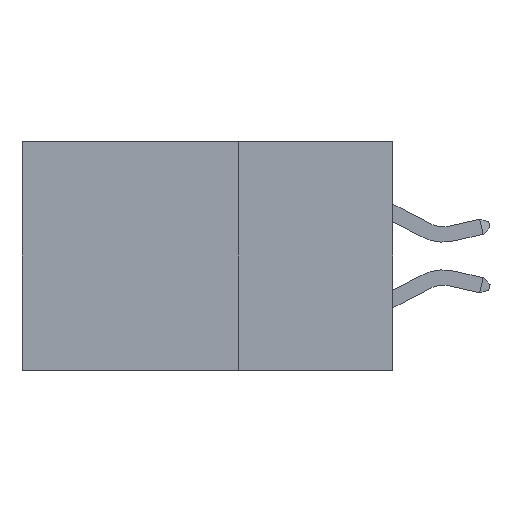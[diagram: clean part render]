
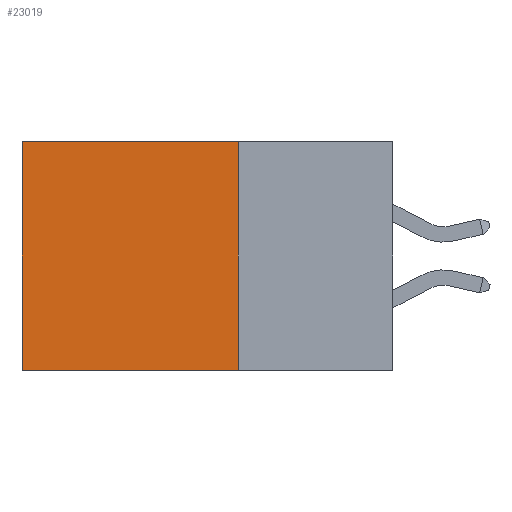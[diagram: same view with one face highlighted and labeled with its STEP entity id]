
A CAD part, left-side view. The second image highlights one B-rep face of the part: STEP entity #23019.
In plain terms, the highlighted planar face has unit normal (-1, 0, 0).
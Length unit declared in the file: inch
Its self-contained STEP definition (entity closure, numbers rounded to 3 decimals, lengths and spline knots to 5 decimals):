
#319 = CARTESIAN_POINT ( 'NONE',  ( 0.2875, 0.6, -0.37 ) ) ;
#680 = ORIENTED_EDGE ( 'NONE', *, *, #13594, .T. ) ;
#1024 = CARTESIAN_POINT ( 'NONE',  ( 0.2875, 0.25, 0. ) ) ;
#2021 = LINE ( 'NONE', #1024, #28720 ) ;
#2973 = EDGE_LOOP ( 'NONE', ( #680, #29762, #11356, #15714 ) ) ;
#3159 = VECTOR ( 'NONE', #13991, 39.37008 ) ;
#4450 = DIRECTION ( 'NONE',  ( 0., 1., 0. ) ) ;
#5563 = VERTEX_POINT ( 'NONE', #319 ) ;
#6186 = DIRECTION ( 'NONE',  ( 0., 0., -1. ) ) ;
#6781 = CARTESIAN_POINT ( 'NONE',  ( 0.2875, 0.25, -0.37 ) ) ;
#6893 = CARTESIAN_POINT ( 'NONE',  ( 0.2875, 0.25, -0.37 ) ) ;
#8074 = LINE ( 'NONE', #29714, #28807 ) ;
#8565 = CARTESIAN_POINT ( 'NONE',  ( 0.2875, 0.25, 0. ) ) ;
#8981 = VERTEX_POINT ( 'NONE', #8565 ) ;
#9592 = LINE ( 'NONE', #6893, #12648 ) ;
#9900 = PLANE ( 'NONE',  #10749 ) ;
#10749 = AXIS2_PLACEMENT_3D ( 'NONE', #19588, #26543, #12347 ) ;
#11356 = ORIENTED_EDGE ( 'NONE', *, *, #23941, .F. ) ;
#12347 = DIRECTION ( 'NONE',  ( 0., 0., -1. ) ) ;
#12648 = VECTOR ( 'NONE', #4450, 39.37008 ) ;
#12972 = FACE_OUTER_BOUND ( 'NONE', #2973, .T. ) ;
#13594 = EDGE_CURVE ( 'NONE', #27870, #5563, #16407, .T. ) ;
#13632 = EDGE_CURVE ( 'NONE', #14733, #5563, #9592, .T. ) ;
#13991 = DIRECTION ( 'NONE',  ( 0., 0., -1. ) ) ;
#14733 = VERTEX_POINT ( 'NONE', #6781 ) ;
#15714 = ORIENTED_EDGE ( 'NONE', *, *, #22500, .T. ) ;
#16407 = LINE ( 'NONE', #23647, #3159 ) ;
#19588 = CARTESIAN_POINT ( 'NONE',  ( 0.2875, 0.25, 0. ) ) ;
#22500 = EDGE_CURVE ( 'NONE', #8981, #27870, #8074, .T. ) ;
#23019 = ADVANCED_FACE ( 'NONE', ( #12972 ), #9900, .F. ) ;
#23647 = CARTESIAN_POINT ( 'NONE',  ( 0.2875, 0.6, 0. ) ) ;
#23941 = EDGE_CURVE ( 'NONE', #8981, #14733, #2021, .T. ) ;
#26543 = DIRECTION ( 'NONE',  ( 1., 0., 0. ) ) ;
#27870 = VERTEX_POINT ( 'NONE', #28608 ) ;
#28608 = CARTESIAN_POINT ( 'NONE',  ( 0.2875, 0.6, 0. ) ) ;
#28720 = VECTOR ( 'NONE', #6186, 39.37008 ) ;
#28807 = VECTOR ( 'NONE', #29819, 39.37008 ) ;
#29714 = CARTESIAN_POINT ( 'NONE',  ( 0.2875, 0.25, 0. ) ) ;
#29762 = ORIENTED_EDGE ( 'NONE', *, *, #13632, .F. ) ;
#29819 = DIRECTION ( 'NONE',  ( 0., 1., 0. ) ) ;
